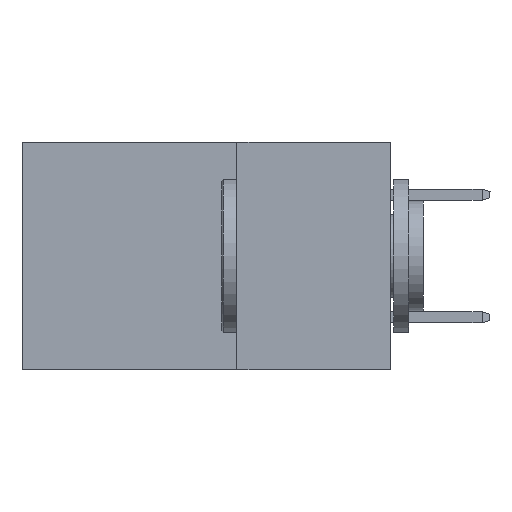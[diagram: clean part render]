
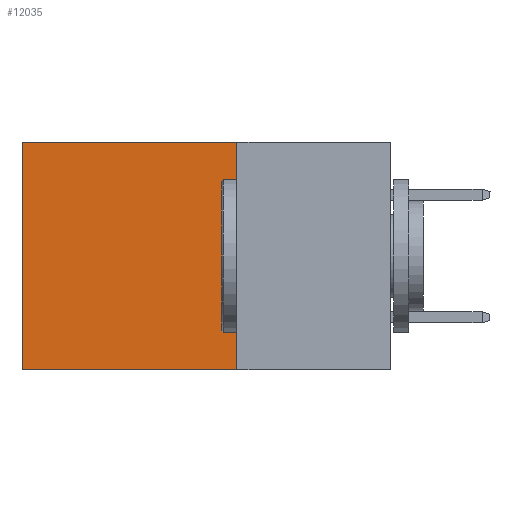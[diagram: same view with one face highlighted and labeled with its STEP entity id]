
A CAD part, left-side view. The second image highlights one B-rep face of the part: STEP entity #12035.
In plain terms, the highlighted planar face has unit normal (-1, 0, 0).
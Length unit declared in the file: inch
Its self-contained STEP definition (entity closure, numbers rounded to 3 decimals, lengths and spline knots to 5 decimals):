
#449 = EDGE_CURVE ( 'NONE', #5749, #5553, #1290, .T. ) ;
#641 = EDGE_CURVE ( 'NONE', #29716, #14981, #14649, .T. ) ;
#870 = DIRECTION ( 'NONE',  ( 0., 1., 0. ) ) ;
#1290 = LINE ( 'NONE', #20303, #6860 ) ;
#1950 = DIRECTION ( 'NONE',  ( 0., 0., -1. ) ) ;
#3810 = CARTESIAN_POINT ( 'NONE',  ( 0.2875, 0.25, 0. ) ) ;
#5248 = DIRECTION ( 'NONE',  ( 0., 0., -1. ) ) ;
#5553 = VERTEX_POINT ( 'NONE', #22606 ) ;
#5749 = VERTEX_POINT ( 'NONE', #9566 ) ;
#6860 = VECTOR ( 'NONE', #870, 39.37008 ) ;
#7446 = DIRECTION ( 'NONE',  ( 0., 0., -1. ) ) ;
#8344 = EDGE_CURVE ( 'NONE', #29716, #5749, #10247, .T. ) ;
#9144 = ORIENTED_EDGE ( 'NONE', *, *, #641, .T. ) ;
#9566 = CARTESIAN_POINT ( 'NONE',  ( 0.2875, 0.25, -0.37 ) ) ;
#10247 = LINE ( 'NONE', #21227, #26977 ) ;
#10721 = CARTESIAN_POINT ( 'NONE',  ( 0.2875, 0.25, 0. ) ) ;
#10744 = ORIENTED_EDGE ( 'NONE', *, *, #8344, .F. ) ;
#11215 = PLANE ( 'NONE',  #21284 ) ;
#11462 = FACE_OUTER_BOUND ( 'NONE', #28101, .T. ) ;
#12035 = ADVANCED_FACE ( 'NONE', ( #11462 ), #11215, .F. ) ;
#12549 = ORIENTED_EDGE ( 'NONE', *, *, #27964, .T. ) ;
#13924 = VECTOR ( 'NONE', #23323, 39.37008 ) ;
#14649 = LINE ( 'NONE', #3810, #13924 ) ;
#14981 = VERTEX_POINT ( 'NONE', #15328 ) ;
#15328 = CARTESIAN_POINT ( 'NONE',  ( 0.2875, 0.6, 0. ) ) ;
#15734 = DIRECTION ( 'NONE',  ( 1., 0., 0. ) ) ;
#20303 = CARTESIAN_POINT ( 'NONE',  ( 0.2875, 0.25, -0.37 ) ) ;
#20419 = VECTOR ( 'NONE', #7446, 39.37008 ) ;
#21049 = CARTESIAN_POINT ( 'NONE',  ( 0.2875, 0.6, 0. ) ) ;
#21227 = CARTESIAN_POINT ( 'NONE',  ( 0.2875, 0.25, 0. ) ) ;
#21284 = AXIS2_PLACEMENT_3D ( 'NONE', #27151, #15734, #1950 ) ;
#22606 = CARTESIAN_POINT ( 'NONE',  ( 0.2875, 0.6, -0.37 ) ) ;
#23323 = DIRECTION ( 'NONE',  ( 0., 1., 0. ) ) ;
#26977 = VECTOR ( 'NONE', #5248, 39.37008 ) ;
#27151 = CARTESIAN_POINT ( 'NONE',  ( 0.2875, 0.25, 0. ) ) ;
#27907 = ORIENTED_EDGE ( 'NONE', *, *, #449, .F. ) ;
#27942 = LINE ( 'NONE', #21049, #20419 ) ;
#27964 = EDGE_CURVE ( 'NONE', #14981, #5553, #27942, .T. ) ;
#28101 = EDGE_LOOP ( 'NONE', ( #12549, #27907, #10744, #9144 ) ) ;
#29716 = VERTEX_POINT ( 'NONE', #10721 ) ;
